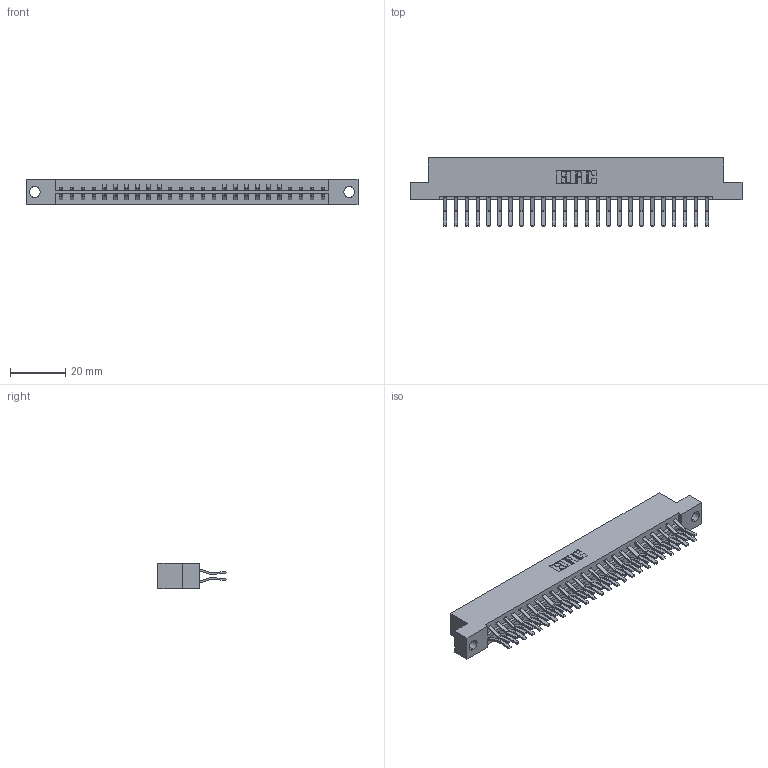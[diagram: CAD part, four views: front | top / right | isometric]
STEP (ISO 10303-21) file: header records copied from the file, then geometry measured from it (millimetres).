
FILE_DESCRIPTION (( 'STEP AP203' ), '1' );
FILE_NAME ('833-050-560-204.STEP', '2020-06-04T18:26:24', ( '' ), ( '' ), 'SwSTEP 2.0', 'SolidWorks 2020', '' );
FILE_SCHEMA (( 'CONFIG_CONTROL_DESIGN' ));
Length unit declared in the file: inch
Products named in the file (3): 833-050-560-204; 833 Part_Flush - .156 Dia - TH; 345-292-001_560 Tail
Assembly tree (51 placements, depth 2):
  833-050-560-204
    833 Part_Flush - .156 Dia - TH
    345-292-001_560 Tail  x50
Bounding box: 120.6 x 24.78 x 9.4 mm (x, y, z)
Volume: 12393.4 mm3; surface area: 15203.7 mm2
Topology: 51 solids, 51 shells, 2814 faces, 8361 edges, 5506 vertices
Faces by surface type: plane 1870, cylinder 944
Entity records: 18373 total; most frequent: CARTESIAN_POINT 3066, ORIENTED_EDGE 3002, DIRECTION 2653, EDGE_CURVE 1501, LINE 1369, VECTOR 1369, VERTEX_POINT 998, AXIS2_PLACEMENT_3D 642
